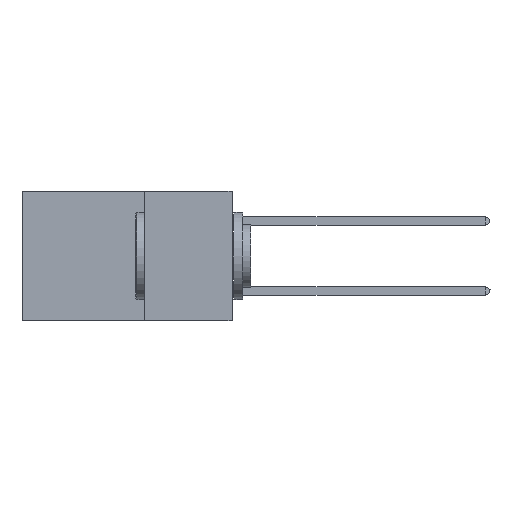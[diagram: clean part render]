
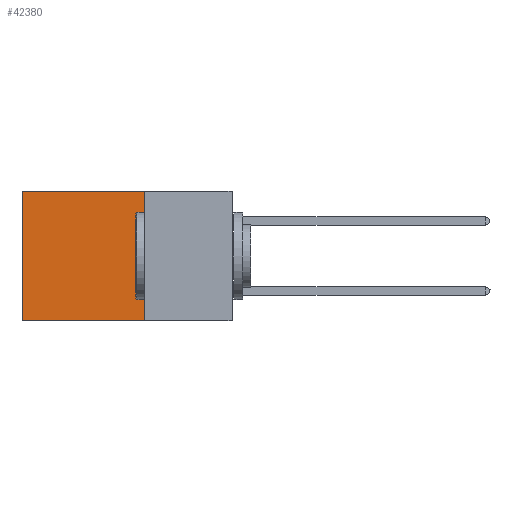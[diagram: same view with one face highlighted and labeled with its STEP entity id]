
A CAD part, left-side view. The second image highlights one B-rep face of the part: STEP entity #42380.
In plain terms, the highlighted planar face has unit normal (-1, 0, 0).
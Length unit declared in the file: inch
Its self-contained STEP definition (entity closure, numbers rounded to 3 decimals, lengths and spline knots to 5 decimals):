
#1801 = CARTESIAN_POINT ( 'NONE',  ( 0.2875, 0.6, 0. ) ) ;
#3244 = VECTOR ( 'NONE', #36398, 39.37008 ) ;
#4399 = EDGE_LOOP ( 'NONE', ( #34787, #41071, #22099, #43679 ) ) ;
#4538 = DIRECTION ( 'NONE',  ( 0., 1., 0. ) ) ;
#4841 = CARTESIAN_POINT ( 'NONE',  ( 0.2875, 0.25, -0.37 ) ) ;
#6290 = CARTESIAN_POINT ( 'NONE',  ( 0.2875, 0.25, -0.37 ) ) ;
#8946 = LINE ( 'NONE', #33633, #29695 ) ;
#9634 = EDGE_CURVE ( 'NONE', #32049, #28788, #13218, .T. ) ;
#10226 = DIRECTION ( 'NONE',  ( 0., 0., -1. ) ) ;
#11390 = VERTEX_POINT ( 'NONE', #25115 ) ;
#13218 = LINE ( 'NONE', #4841, #35058 ) ;
#15418 = VERTEX_POINT ( 'NONE', #1801 ) ;
#16213 = VECTOR ( 'NONE', #19769, 39.37008 ) ;
#19769 = DIRECTION ( 'NONE',  ( 0., 1., 0. ) ) ;
#20768 = LINE ( 'NONE', #32840, #3244 ) ;
#22099 = ORIENTED_EDGE ( 'NONE', *, *, #43522, .F. ) ;
#23909 = CARTESIAN_POINT ( 'NONE',  ( 0.2875, 0.25, 0. ) ) ;
#25031 = AXIS2_PLACEMENT_3D ( 'NONE', #23909, #33873, #10226 ) ;
#25115 = CARTESIAN_POINT ( 'NONE',  ( 0.2875, 0.25, 0. ) ) ;
#25284 = LINE ( 'NONE', #29904, #16213 ) ;
#25469 = CARTESIAN_POINT ( 'NONE',  ( 0.2875, 0.6, -0.37 ) ) ;
#28788 = VERTEX_POINT ( 'NONE', #25469 ) ;
#29695 = VECTOR ( 'NONE', #40030, 39.37008 ) ;
#29904 = CARTESIAN_POINT ( 'NONE',  ( 0.2875, 0.25, 0. ) ) ;
#30589 = PLANE ( 'NONE',  #25031 ) ;
#30733 = FACE_OUTER_BOUND ( 'NONE', #4399, .T. ) ;
#32049 = VERTEX_POINT ( 'NONE', #6290 ) ;
#32840 = CARTESIAN_POINT ( 'NONE',  ( 0.2875, 0.6, 0. ) ) ;
#33356 = EDGE_CURVE ( 'NONE', #15418, #28788, #20768, .T. ) ;
#33633 = CARTESIAN_POINT ( 'NONE',  ( 0.2875, 0.25, 0. ) ) ;
#33873 = DIRECTION ( 'NONE',  ( 1., 0., 0. ) ) ;
#34787 = ORIENTED_EDGE ( 'NONE', *, *, #33356, .T. ) ;
#35058 = VECTOR ( 'NONE', #4538, 39.37008 ) ;
#36398 = DIRECTION ( 'NONE',  ( 0., 0., -1. ) ) ;
#37235 = EDGE_CURVE ( 'NONE', #11390, #15418, #25284, .T. ) ;
#40030 = DIRECTION ( 'NONE',  ( 0., 0., -1. ) ) ;
#41071 = ORIENTED_EDGE ( 'NONE', *, *, #9634, .F. ) ;
#42380 = ADVANCED_FACE ( 'NONE', ( #30733 ), #30589, .F. ) ;
#43522 = EDGE_CURVE ( 'NONE', #11390, #32049, #8946, .T. ) ;
#43679 = ORIENTED_EDGE ( 'NONE', *, *, #37235, .T. ) ;
